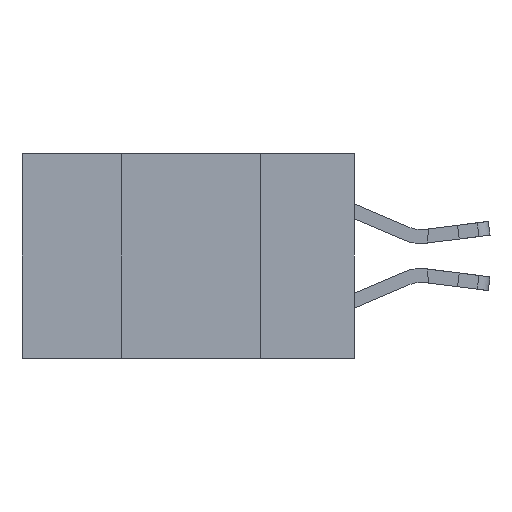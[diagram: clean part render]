
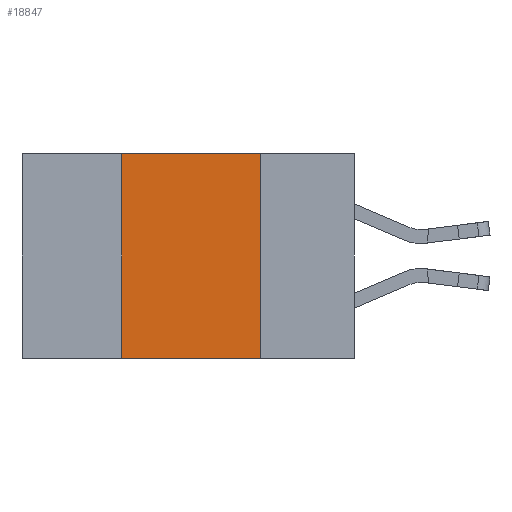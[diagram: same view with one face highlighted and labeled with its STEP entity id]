
A CAD part, left-side view. The second image highlights one B-rep face of the part: STEP entity #18847.
In plain terms, the highlighted planar face has unit normal (-1, 0, 0).
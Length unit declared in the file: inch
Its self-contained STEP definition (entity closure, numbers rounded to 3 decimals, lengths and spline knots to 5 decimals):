
#248 = FACE_OUTER_BOUND ( 'NONE', #1574, .T. ) ;
#952 = DIRECTION ( 'NONE',  ( 0., -1., 0. ) ) ;
#1318 = VERTEX_POINT ( 'NONE', #3052 ) ;
#1574 = EDGE_LOOP ( 'NONE', ( #16058, #12559, #6160, #14605 ) ) ;
#2394 = CARTESIAN_POINT ( 'NONE',  ( 0., 0.6, 0. ) ) ;
#2586 = VERTEX_POINT ( 'NONE', #5960 ) ;
#2672 = LINE ( 'NONE', #19478, #16299 ) ;
#2765 = VECTOR ( 'NONE', #14128, 39.37008 ) ;
#3052 = CARTESIAN_POINT ( 'NONE',  ( 0., 0.17, 0. ) ) ;
#5023 = CARTESIAN_POINT ( 'NONE',  ( 0., 0.6, 0. ) ) ;
#5136 = LINE ( 'NONE', #15641, #20779 ) ;
#5483 = CARTESIAN_POINT ( 'NONE',  ( 0., 0.17, -0.37 ) ) ;
#5871 = EDGE_CURVE ( 'NONE', #11833, #2586, #5136, .T. ) ;
#5960 = CARTESIAN_POINT ( 'NONE',  ( 0., 0.17, -0.37 ) ) ;
#6160 = ORIENTED_EDGE ( 'NONE', *, *, #12564, .F. ) ;
#6785 = DIRECTION ( 'NONE',  ( 0., 0., -1. ) ) ;
#6989 = DIRECTION ( 'NONE',  ( 1., 0., 0. ) ) ;
#7385 = EDGE_CURVE ( 'NONE', #1318, #2586, #14751, .T. ) ;
#10048 = CARTESIAN_POINT ( 'NONE',  ( 0., 0.42, -0.37 ) ) ;
#10090 = VERTEX_POINT ( 'NONE', #17724 ) ;
#11833 = VERTEX_POINT ( 'NONE', #10048 ) ;
#11884 = PLANE ( 'NONE',  #14366 ) ;
#12559 = ORIENTED_EDGE ( 'NONE', *, *, #16462, .F. ) ;
#12564 = EDGE_CURVE ( 'NONE', #11833, #10090, #2672, .T. ) ;
#12572 = LINE ( 'NONE', #2394, #15639 ) ;
#14128 = DIRECTION ( 'NONE',  ( 0., 0., -1. ) ) ;
#14366 = AXIS2_PLACEMENT_3D ( 'NONE', #5023, #6989, #6785 ) ;
#14605 = ORIENTED_EDGE ( 'NONE', *, *, #5871, .T. ) ;
#14751 = LINE ( 'NONE', #5483, #2765 ) ;
#15639 = VECTOR ( 'NONE', #952, 39.37008 ) ;
#15641 = CARTESIAN_POINT ( 'NONE',  ( 0., 0.6, -0.37 ) ) ;
#16058 = ORIENTED_EDGE ( 'NONE', *, *, #7385, .F. ) ;
#16299 = VECTOR ( 'NONE', #21146, 39.37008 ) ;
#16462 = EDGE_CURVE ( 'NONE', #10090, #1318, #12572, .T. ) ;
#17724 = CARTESIAN_POINT ( 'NONE',  ( 0., 0.42, 0. ) ) ;
#18847 = ADVANCED_FACE ( 'NONE', ( #248 ), #11884, .F. ) ;
#19053 = DIRECTION ( 'NONE',  ( 0., -1., 0. ) ) ;
#19478 = CARTESIAN_POINT ( 'NONE',  ( 0., 0.42, -0.37 ) ) ;
#20779 = VECTOR ( 'NONE', #19053, 39.37008 ) ;
#21146 = DIRECTION ( 'NONE',  ( 0., 0., 1. ) ) ;
